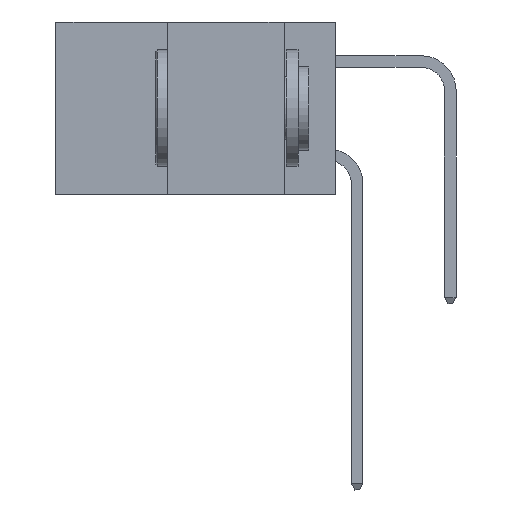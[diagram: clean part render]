
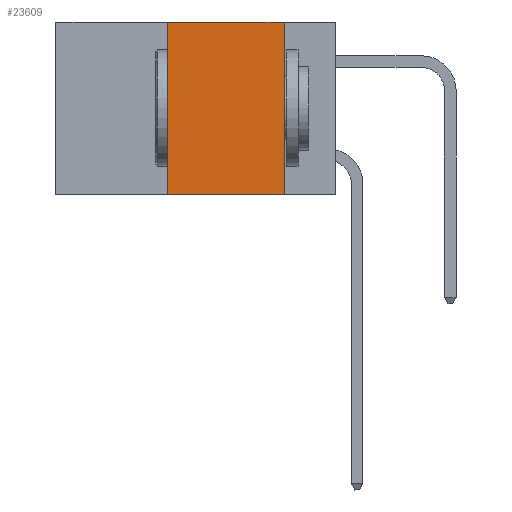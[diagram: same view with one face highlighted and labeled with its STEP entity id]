
A CAD part, left-side view. The second image highlights one B-rep face of the part: STEP entity #23609.
In plain terms, the highlighted planar face has unit normal (-1, 0, 0).
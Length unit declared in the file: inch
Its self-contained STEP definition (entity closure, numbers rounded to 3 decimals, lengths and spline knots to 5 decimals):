
#1053 = ORIENTED_EDGE ( 'NONE', *, *, #23700, .T. ) ;
#1154 = DIRECTION ( 'NONE',  ( 0., 0., -1. ) ) ;
#2858 = PLANE ( 'NONE',  #20046 ) ;
#3443 = CARTESIAN_POINT ( 'NONE',  ( 0., 0.36, -0.37 ) ) ;
#3604 = CARTESIAN_POINT ( 'NONE',  ( 0., 0.36, 0. ) ) ;
#3836 = CARTESIAN_POINT ( 'NONE',  ( 0., 0.36, 0. ) ) ;
#3878 = ORIENTED_EDGE ( 'NONE', *, *, #22005, .F. ) ;
#4576 = LINE ( 'NONE', #7046, #14470 ) ;
#6523 = EDGE_CURVE ( 'NONE', #24004, #24730, #23415, .T. ) ;
#6873 = CARTESIAN_POINT ( 'NONE',  ( 0., 0.6, 0. ) ) ;
#7046 = CARTESIAN_POINT ( 'NONE',  ( 0., 0.6, -0.37 ) ) ;
#7947 = ORIENTED_EDGE ( 'NONE', *, *, #18408, .F. ) ;
#8111 = VECTOR ( 'NONE', #19419, 39.37008 ) ;
#8871 = DIRECTION ( 'NONE',  ( 0., 0., -1. ) ) ;
#9034 = DIRECTION ( 'NONE',  ( 0., -1., 0. ) ) ;
#11684 = VECTOR ( 'NONE', #1154, 39.37008 ) ;
#12965 = CARTESIAN_POINT ( 'NONE',  ( 0., 0.11, -0.37 ) ) ;
#14470 = VECTOR ( 'NONE', #9034, 39.37008 ) ;
#15470 = DIRECTION ( 'NONE',  ( 0., 0., 1. ) ) ;
#15805 = VERTEX_POINT ( 'NONE', #19302 ) ;
#17455 = CARTESIAN_POINT ( 'NONE',  ( 0., 0.6, 0. ) ) ;
#17739 = EDGE_LOOP ( 'NONE', ( #7947, #3878, #20261, #1053 ) ) ;
#17952 = LINE ( 'NONE', #17455, #8111 ) ;
#18181 = VECTOR ( 'NONE', #15470, 39.37008 ) ;
#18386 = VERTEX_POINT ( 'NONE', #12965 ) ;
#18408 = EDGE_CURVE ( 'NONE', #15805, #18386, #18787, .T. ) ;
#18787 = LINE ( 'NONE', #20973, #11684 ) ;
#19302 = CARTESIAN_POINT ( 'NONE',  ( 0., 0.11, 0. ) ) ;
#19419 = DIRECTION ( 'NONE',  ( 0., -1., 0. ) ) ;
#20046 = AXIS2_PLACEMENT_3D ( 'NONE', #6873, #20649, #8871 ) ;
#20261 = ORIENTED_EDGE ( 'NONE', *, *, #6523, .F. ) ;
#20649 = DIRECTION ( 'NONE',  ( 1., 0., 0. ) ) ;
#20973 = CARTESIAN_POINT ( 'NONE',  ( 0., 0.11, 0. ) ) ;
#21575 = FACE_OUTER_BOUND ( 'NONE', #17739, .T. ) ;
#22005 = EDGE_CURVE ( 'NONE', #24730, #15805, #17952, .T. ) ;
#23415 = LINE ( 'NONE', #3604, #18181 ) ;
#23609 = ADVANCED_FACE ( 'NONE', ( #21575 ), #2858, .F. ) ;
#23700 = EDGE_CURVE ( 'NONE', #24004, #18386, #4576, .T. ) ;
#24004 = VERTEX_POINT ( 'NONE', #3443 ) ;
#24730 = VERTEX_POINT ( 'NONE', #3836 ) ;
